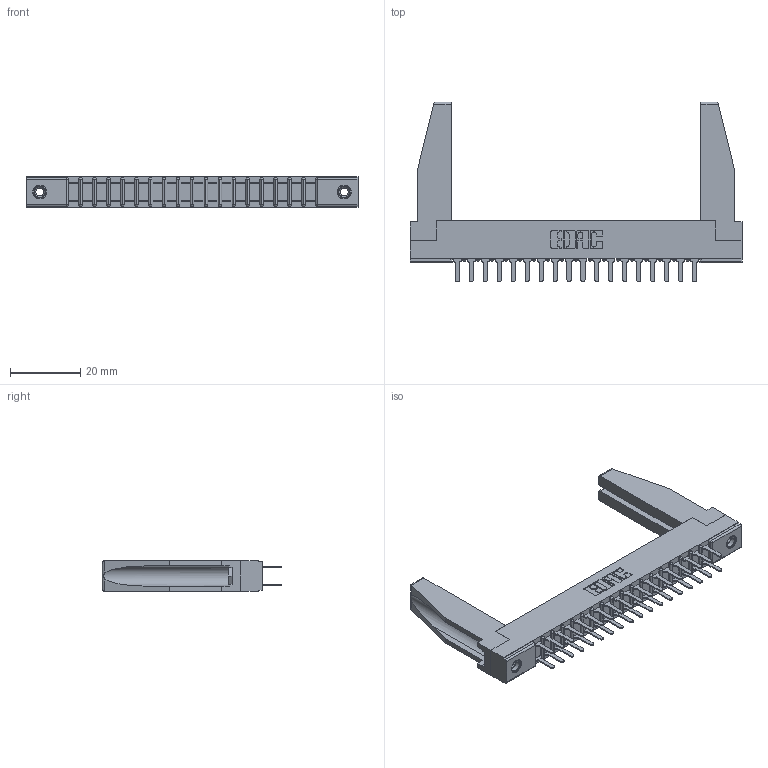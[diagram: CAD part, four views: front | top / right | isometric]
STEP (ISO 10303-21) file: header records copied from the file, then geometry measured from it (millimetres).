
FILE_DESCRIPTION (( 'STEP AP203' ), '1' );
FILE_NAME ('357-036-420-278.STEP', '2020-10-03T17:17:19', ( '' ), ( '' ), 'SwSTEP 2.0', 'SolidWorks 2020', '' );
FILE_SCHEMA (( 'CONFIG_CONTROL_DESIGN' ));
Length unit declared in the file: inch
Products named in the file (5): 357-036-420-278; 307 Part_.156 Dia Mounting Holes; 307-220-078; 307-290-001_520; 345-250-001_345-250-001-102
Assembly tree (41 placements, depth 2):
  357-036-420-278
    307 Part_.156 Dia Mounting Holes
    307-290-001_520  x36
    307-220-078  x2
    345-250-001_345-250-001-102  x2
Bounding box: 94.34 x 51.13 x 8.71 mm (x, y, z)
Volume: 10190.7 mm3; surface area: 14660.4 mm2
Topology: 41 solids, 41 shells, 1923 faces, 5333 edges, 3446 vertices
Faces by surface type: plane 1270, cylinder 599, sphere 38, cone 12, torus 4
Entity records: 21373 total; most frequent: CARTESIAN_POINT 3512, ORIENTED_EDGE 3436, DIRECTION 3404, EDGE_CURVE 1718, LINE 1312, VECTOR 1312, VERTEX_POINT 1112, AXIS2_PLACEMENT_3D 1046
